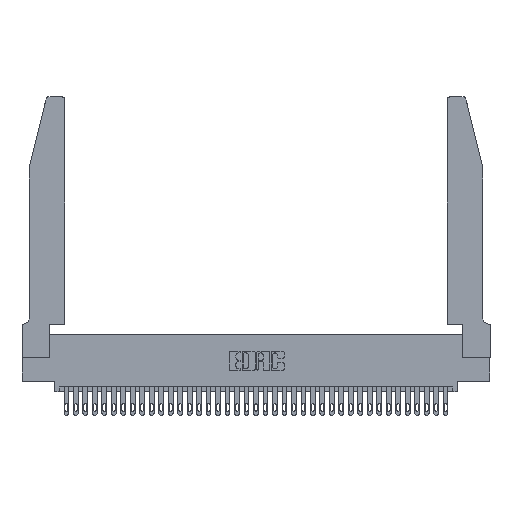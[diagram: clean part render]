
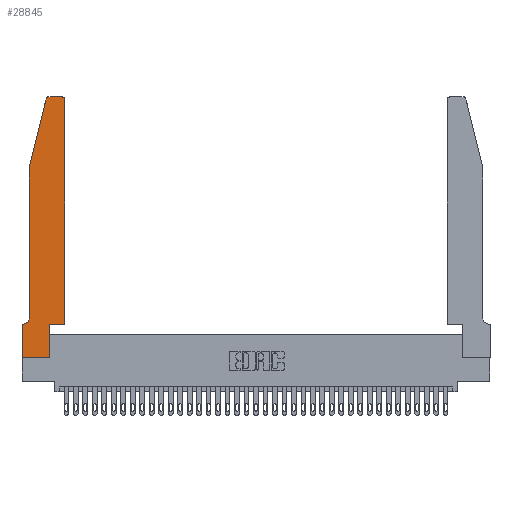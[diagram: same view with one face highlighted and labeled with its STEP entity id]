
A CAD part, top view. The second image highlights one B-rep face of the part: STEP entity #28845.
In plain terms, the highlighted planar face has unit normal (0, 0, 1).
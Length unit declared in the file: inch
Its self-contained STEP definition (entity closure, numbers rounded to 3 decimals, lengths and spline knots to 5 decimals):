
#802 = ORIENTED_EDGE ( 'NONE', *, *, #18313, .T. ) ;
#894 = DIRECTION ( 'NONE',  ( 0., 0., 1. ) ) ;
#1084 = LINE ( 'NONE', #24343, #7405 ) ;
#1147 = CARTESIAN_POINT ( 'NONE',  ( 0.4205, 2.72, 0.37 ) ) ;
#1153 = VERTEX_POINT ( 'NONE', #34007 ) ;
#1201 = VERTEX_POINT ( 'NONE', #15489 ) ;
#1442 = CARTESIAN_POINT ( 'NONE',  ( 0.4505, 2.72, 0.37 ) ) ;
#1893 = CARTESIAN_POINT ( 'NONE',  ( 0.284, 2.75, 0.37 ) ) ;
#2090 = CARTESIAN_POINT ( 'NONE',  ( 0.0055, 0.42, 0.37 ) ) ;
#2419 = CARTESIAN_POINT ( 'NONE',  ( 0.0755, 2., 0.37 ) ) ;
#2766 = EDGE_CURVE ( 'NONE', #13231, #28739, #8730, .T. ) ;
#3166 = FACE_OUTER_BOUND ( 'NONE', #17565, .T. ) ;
#3886 = VECTOR ( 'NONE', #25397, 39.37008 ) ;
#3973 = CARTESIAN_POINT ( 'NONE',  ( 0., 0.35, 0.37 ) ) ;
#4223 = CARTESIAN_POINT ( 'NONE',  ( 0.2605, 2.75, 0.37 ) ) ;
#5218 = EDGE_CURVE ( 'NONE', #10896, #1201, #32328, .T. ) ;
#5268 = LINE ( 'NONE', #26617, #6979 ) ;
#6042 = CIRCLE ( 'NONE', #6980, 0.03 ) ;
#6656 = CARTESIAN_POINT ( 'NONE',  ( 0.0755, 2., 0.37 ) ) ;
#6736 = LINE ( 'NONE', #12684, #9924 ) ;
#6979 = VECTOR ( 'NONE', #29329, 39.37008 ) ;
#6980 = AXIS2_PLACEMENT_3D ( 'NONE', #1147, #894, #12106 ) ;
#7379 = DIRECTION ( 'NONE',  ( 1., 0., 0. ) ) ;
#7405 = VECTOR ( 'NONE', #11941, 39.37008 ) ;
#7529 = EDGE_CURVE ( 'NONE', #1201, #13231, #25055, .T. ) ;
#8633 = VECTOR ( 'NONE', #30072, 39.37008 ) ;
#8709 = ORIENTED_EDGE ( 'NONE', *, *, #14177, .T. ) ;
#8730 = LINE ( 'NONE', #6656, #11002 ) ;
#8861 = ORIENTED_EDGE ( 'NONE', *, *, #13470, .T. ) ;
#9167 = EDGE_CURVE ( 'NONE', #10808, #34206, #15742, .T. ) ;
#9492 = DIRECTION ( 'NONE',  ( 0., 0., 1. ) ) ;
#9834 = CARTESIAN_POINT ( 'NONE',  ( 0., 0., 0.37 ) ) ;
#9924 = VECTOR ( 'NONE', #15694, 39.37008 ) ;
#10469 = DIRECTION ( 'NONE',  ( 0., 0., -1. ) ) ;
#10720 = CARTESIAN_POINT ( 'NONE',  ( 0.0055, 0.35, 0.37 ) ) ;
#10808 = VERTEX_POINT ( 'NONE', #13989 ) ;
#10896 = VERTEX_POINT ( 'NONE', #1893 ) ;
#11002 = VECTOR ( 'NONE', #26645, 39.37008 ) ;
#11043 = CARTESIAN_POINT ( 'NONE',  ( 0.4505, 0.35, 0.37 ) ) ;
#11941 = DIRECTION ( 'NONE',  ( 0., 1., 0. ) ) ;
#12101 = DIRECTION ( 'NONE',  ( 1., 0., 0. ) ) ;
#12106 = DIRECTION ( 'NONE',  ( 1., 0., 0. ) ) ;
#12303 = CIRCLE ( 'NONE', #21148, 0.07 ) ;
#12684 = CARTESIAN_POINT ( 'NONE',  ( 0.4505, 0.35, 0.37 ) ) ;
#12774 = ORIENTED_EDGE ( 'NONE', *, *, #14328, .T. ) ;
#13231 = VERTEX_POINT ( 'NONE', #16403 ) ;
#13470 = EDGE_CURVE ( 'NONE', #28580, #1153, #21344, .T. ) ;
#13812 = EDGE_CURVE ( 'NONE', #31533, #10808, #1084, .T. ) ;
#13978 = AXIS2_PLACEMENT_3D ( 'NONE', #3973, #9492, #23937 ) ;
#13989 = CARTESIAN_POINT ( 'NONE',  ( 0.2865, 0.35, 0.37 ) ) ;
#14177 = EDGE_CURVE ( 'NONE', #14962, #33260, #6042, .T. ) ;
#14328 = EDGE_CURVE ( 'NONE', #28739, #36451, #12303, .T. ) ;
#14962 = VERTEX_POINT ( 'NONE', #1442 ) ;
#15489 = CARTESIAN_POINT ( 'NONE',  ( 0.25487, 2.72718, 0.37 ) ) ;
#15694 = DIRECTION ( 'NONE',  ( 0., 1., 0. ) ) ;
#15742 = LINE ( 'NONE', #11043, #23408 ) ;
#15944 = VECTOR ( 'NONE', #19487, 39.37008 ) ;
#16298 = DIRECTION ( 'NONE',  ( 0., 0., 1. ) ) ;
#16403 = CARTESIAN_POINT ( 'NONE',  ( 0.0755, 2., 0.37 ) ) ;
#16621 = CARTESIAN_POINT ( 'NONE',  ( 0., 0., 0.37 ) ) ;
#16819 = CARTESIAN_POINT ( 'NONE',  ( 0.4205, 2.75, 0.37 ) ) ;
#17565 = EDGE_LOOP ( 'NONE', ( #20502, #34241, #18806, #28378, #12774, #25715, #8861, #802, #18099, #20541, #24311, #8709 ) ) ;
#17704 = VECTOR ( 'NONE', #12101, 39.37008 ) ;
#18099 = ORIENTED_EDGE ( 'NONE', *, *, #13812, .T. ) ;
#18145 = PLANE ( 'NONE',  #13978 ) ;
#18313 = EDGE_CURVE ( 'NONE', #1153, #31533, #22242, .T. ) ;
#18806 = ORIENTED_EDGE ( 'NONE', *, *, #7529, .T. ) ;
#19487 = DIRECTION ( 'NONE',  ( 0., -1., 0. ) ) ;
#20223 = EDGE_CURVE ( 'NONE', #33260, #10896, #21092, .T. ) ;
#20264 = EDGE_CURVE ( 'NONE', #34206, #14962, #6736, .T. ) ;
#20502 = ORIENTED_EDGE ( 'NONE', *, *, #20223, .T. ) ;
#20541 = ORIENTED_EDGE ( 'NONE', *, *, #9167, .T. ) ;
#21092 = LINE ( 'NONE', #4223, #8633 ) ;
#21148 = AXIS2_PLACEMENT_3D ( 'NONE', #2090, #10469, #30296 ) ;
#21344 = LINE ( 'NONE', #16621, #15944 ) ;
#22242 = LINE ( 'NONE', #9834, #17704 ) ;
#23408 = VECTOR ( 'NONE', #24826, 39.37008 ) ;
#23937 = DIRECTION ( 'NONE',  ( 1., 0., 0. ) ) ;
#24311 = ORIENTED_EDGE ( 'NONE', *, *, #20264, .T. ) ;
#24343 = CARTESIAN_POINT ( 'NONE',  ( 0.2865, 0.35, 0.37 ) ) ;
#24826 = DIRECTION ( 'NONE',  ( 1., 0., 0. ) ) ;
#25055 = LINE ( 'NONE', #2419, #3886 ) ;
#25397 = DIRECTION ( 'NONE',  ( -0.239, -0.971, 0. ) ) ;
#25715 = ORIENTED_EDGE ( 'NONE', *, *, #30910, .T. ) ;
#26015 = CARTESIAN_POINT ( 'NONE',  ( 0., 0.35, 0.37 ) ) ;
#26468 = CARTESIAN_POINT ( 'NONE',  ( 0.0755, 0.42, 0.37 ) ) ;
#26617 = CARTESIAN_POINT ( 'NONE',  ( 0.0755, 0.35, 0.37 ) ) ;
#26645 = DIRECTION ( 'NONE',  ( 0., -1., 0. ) ) ;
#28378 = ORIENTED_EDGE ( 'NONE', *, *, #2766, .T. ) ;
#28580 = VERTEX_POINT ( 'NONE', #26015 ) ;
#28739 = VERTEX_POINT ( 'NONE', #26468 ) ;
#28845 = ADVANCED_FACE ( 'NONE', ( #3166 ), #18145, .T. ) ;
#28958 = CARTESIAN_POINT ( 'NONE',  ( 0.2865, 0., 0.37 ) ) ;
#29329 = DIRECTION ( 'NONE',  ( -1., 0., 0. ) ) ;
#30072 = DIRECTION ( 'NONE',  ( -1., 0., 0. ) ) ;
#30296 = DIRECTION ( 'NONE',  ( -1., 0., 0. ) ) ;
#30910 = EDGE_CURVE ( 'NONE', #36451, #28580, #5268, .T. ) ;
#31533 = VERTEX_POINT ( 'NONE', #28958 ) ;
#31902 = CARTESIAN_POINT ( 'NONE',  ( 0.4505, 0.35, 0.37 ) ) ;
#32328 = CIRCLE ( 'NONE', #34244, 0.03 ) ;
#33260 = VERTEX_POINT ( 'NONE', #16819 ) ;
#34007 = CARTESIAN_POINT ( 'NONE',  ( 0., 0., 0.37 ) ) ;
#34206 = VERTEX_POINT ( 'NONE', #31902 ) ;
#34241 = ORIENTED_EDGE ( 'NONE', *, *, #5218, .T. ) ;
#34244 = AXIS2_PLACEMENT_3D ( 'NONE', #35971, #16298, #7379 ) ;
#35971 = CARTESIAN_POINT ( 'NONE',  ( 0.284, 2.72, 0.37 ) ) ;
#36451 = VERTEX_POINT ( 'NONE', #10720 ) ;
